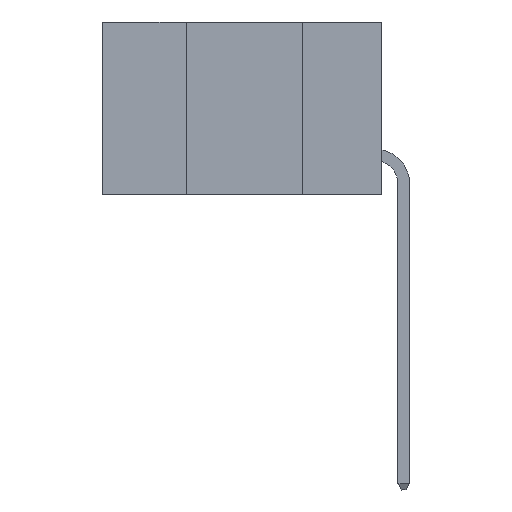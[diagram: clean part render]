
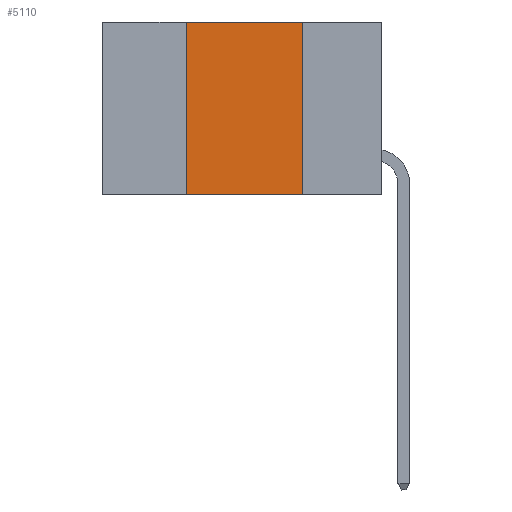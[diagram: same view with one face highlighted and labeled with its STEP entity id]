
A CAD part, left-side view. The second image highlights one B-rep face of the part: STEP entity #5110.
In plain terms, the highlighted planar face has unit normal (-1, 0, 0).
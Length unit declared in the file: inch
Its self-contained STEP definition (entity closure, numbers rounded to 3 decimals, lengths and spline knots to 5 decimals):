
#370 = EDGE_CURVE ( 'NONE', #16944, #13117, #19364, .T. ) ;
#845 = DIRECTION ( 'NONE',  ( 0., 0., 1. ) ) ;
#1119 = CARTESIAN_POINT ( 'NONE',  ( 0., 0.42, -0.37 ) ) ;
#3466 = DIRECTION ( 'NONE',  ( 0., -1., 0. ) ) ;
#3767 = EDGE_CURVE ( 'NONE', #19174, #18190, #19426, .T. ) ;
#5110 = ADVANCED_FACE ( 'NONE', ( #6317 ), #17304, .F. ) ;
#5969 = CARTESIAN_POINT ( 'NONE',  ( 0., 0.6, 0. ) ) ;
#6317 = FACE_OUTER_BOUND ( 'NONE', #13639, .T. ) ;
#6322 = ORIENTED_EDGE ( 'NONE', *, *, #9713, .F. ) ;
#6541 = DIRECTION ( 'NONE',  ( 0., 0., -1. ) ) ;
#7671 = CARTESIAN_POINT ( 'NONE',  ( 0., 0.6, 0. ) ) ;
#7981 = CARTESIAN_POINT ( 'NONE',  ( 0., 0.42, 0. ) ) ;
#9713 = EDGE_CURVE ( 'NONE', #13117, #18190, #20334, .T. ) ;
#9838 = CARTESIAN_POINT ( 'NONE',  ( 0., 0.17, 0. ) ) ;
#9977 = DIRECTION ( 'NONE',  ( 0., 0., -1. ) ) ;
#10659 = VECTOR ( 'NONE', #3466, 39.37008 ) ;
#10958 = DIRECTION ( 'NONE',  ( 1., 0., 0. ) ) ;
#11191 = CARTESIAN_POINT ( 'NONE',  ( 0., 0.17, 0. ) ) ;
#12250 = DIRECTION ( 'NONE',  ( 0., -1., 0. ) ) ;
#13087 = CARTESIAN_POINT ( 'NONE',  ( 0., 0.17, -0.37 ) ) ;
#13117 = VERTEX_POINT ( 'NONE', #11191 ) ;
#13138 = AXIS2_PLACEMENT_3D ( 'NONE', #5969, #10958, #9977 ) ;
#13639 = EDGE_LOOP ( 'NONE', ( #6322, #18704, #15063, #19206 ) ) ;
#14132 = EDGE_CURVE ( 'NONE', #19174, #16944, #19278, .T. ) ;
#14460 = VECTOR ( 'NONE', #845, 39.37008 ) ;
#15063 = ORIENTED_EDGE ( 'NONE', *, *, #14132, .F. ) ;
#15112 = VECTOR ( 'NONE', #12250, 39.37008 ) ;
#15530 = VECTOR ( 'NONE', #6541, 39.37008 ) ;
#16944 = VERTEX_POINT ( 'NONE', #7981 ) ;
#17304 = PLANE ( 'NONE',  #13138 ) ;
#18190 = VERTEX_POINT ( 'NONE', #13087 ) ;
#18704 = ORIENTED_EDGE ( 'NONE', *, *, #370, .F. ) ;
#19174 = VERTEX_POINT ( 'NONE', #1119 ) ;
#19206 = ORIENTED_EDGE ( 'NONE', *, *, #3767, .T. ) ;
#19278 = LINE ( 'NONE', #20525, #14460 ) ;
#19364 = LINE ( 'NONE', #7671, #10659 ) ;
#19426 = LINE ( 'NONE', #21214, #15112 ) ;
#20334 = LINE ( 'NONE', #9838, #15530 ) ;
#20525 = CARTESIAN_POINT ( 'NONE',  ( 0., 0.42, 0. ) ) ;
#21214 = CARTESIAN_POINT ( 'NONE',  ( 0., 0.6, -0.37 ) ) ;
